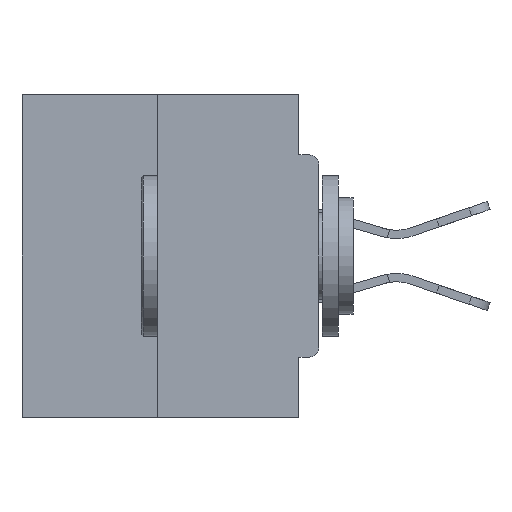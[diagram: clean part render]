
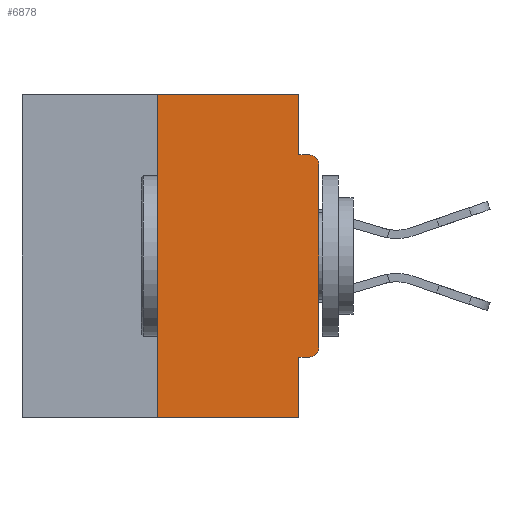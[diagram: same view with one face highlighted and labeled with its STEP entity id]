
A CAD part, left-side view. The second image highlights one B-rep face of the part: STEP entity #6878.
In plain terms, the highlighted planar face has unit normal (-1, 0, 0).
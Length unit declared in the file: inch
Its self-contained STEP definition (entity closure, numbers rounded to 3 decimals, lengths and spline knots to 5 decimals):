
#933 = DIRECTION ( 'NONE',  ( 0., 0., -1. ) ) ;
#1001 = EDGE_CURVE ( 'NONE', #25454, #25395, #29724, .T. ) ;
#1722 = CARTESIAN_POINT ( 'NONE',  ( 0., 0.25, -0.5 ) ) ;
#2146 = ORIENTED_EDGE ( 'NONE', *, *, #30901, .F. ) ;
#3434 = CARTESIAN_POINT ( 'NONE',  ( 0., 0.031, -0.4065 ) ) ;
#4298 = EDGE_LOOP ( 'NONE', ( #2146, #37162, #21792, #23008, #35223, #9632, #7834, #28525, #21918, #13976 ) ) ;
#4309 = DIRECTION ( 'NONE',  ( 0., 0., 1. ) ) ;
#4375 = CARTESIAN_POINT ( 'NONE',  ( 0., 0.25, 0. ) ) ;
#4408 = VERTEX_POINT ( 'NONE', #17975 ) ;
#4445 = EDGE_CURVE ( 'NONE', #8649, #29275, #18057, .T. ) ;
#5433 = LINE ( 'NONE', #18613, #16740 ) ;
#6863 = DIRECTION ( 'NONE',  ( 0., 0., -1. ) ) ;
#6878 = ADVANCED_FACE ( 'NONE', ( #32872 ), #21209, .F. ) ;
#7069 = VECTOR ( 'NONE', #36921, 39.37008 ) ;
#7736 = EDGE_CURVE ( 'NONE', #29275, #28448, #27808, .T. ) ;
#7834 = ORIENTED_EDGE ( 'NONE', *, *, #4445, .T. ) ;
#8486 = LINE ( 'NONE', #9154, #25221 ) ;
#8614 = EDGE_CURVE ( 'NONE', #33012, #25261, #8486, .T. ) ;
#8649 = VERTEX_POINT ( 'NONE', #24083 ) ;
#9154 = CARTESIAN_POINT ( 'NONE',  ( 0., 0., -0.4065 ) ) ;
#9389 = CARTESIAN_POINT ( 'NONE',  ( 0., 0.015, -0.1085 ) ) ;
#9483 = LINE ( 'NONE', #33448, #35346 ) ;
#9632 = ORIENTED_EDGE ( 'NONE', *, *, #24973, .T. ) ;
#10606 = AXIS2_PLACEMENT_3D ( 'NONE', #9389, #29421, #32572 ) ;
#11054 = CARTESIAN_POINT ( 'NONE',  ( 0., 0.25, 0. ) ) ;
#11747 = VECTOR ( 'NONE', #4309, 39.37008 ) ;
#11888 = VECTOR ( 'NONE', #32678, 39.37008 ) ;
#13976 = ORIENTED_EDGE ( 'NONE', *, *, #22977, .F. ) ;
#14160 = CARTESIAN_POINT ( 'NONE',  ( 0., 0.031, -0.5 ) ) ;
#14330 = DIRECTION ( 'NONE',  ( 0., -1., 0. ) ) ;
#15094 = CARTESIAN_POINT ( 'NONE',  ( 0., 0.46, 0. ) ) ;
#15231 = VERTEX_POINT ( 'NONE', #4375 ) ;
#16740 = VECTOR ( 'NONE', #6863, 39.37008 ) ;
#17073 = CARTESIAN_POINT ( 'NONE',  ( 0., 0.015, -0.0935 ) ) ;
#17439 = VECTOR ( 'NONE', #22399, 39.37008 ) ;
#17901 = DIRECTION ( 'NONE',  ( 0., 1., 0. ) ) ;
#17975 = CARTESIAN_POINT ( 'NONE',  ( 0., 0.031, 0. ) ) ;
#18057 = LINE ( 'NONE', #36102, #11747 ) ;
#18613 = CARTESIAN_POINT ( 'NONE',  ( 0., 0.031, 0. ) ) ;
#19743 = VERTEX_POINT ( 'NONE', #37379 ) ;
#21209 = PLANE ( 'NONE',  #28307 ) ;
#21332 = CARTESIAN_POINT ( 'NONE',  ( 0., 0.46, 0. ) ) ;
#21459 = DIRECTION ( 'NONE',  ( 0., 0., -1. ) ) ;
#21792 = ORIENTED_EDGE ( 'NONE', *, *, #1001, .T. ) ;
#21918 = ORIENTED_EDGE ( 'NONE', *, *, #28853, .F. ) ;
#22145 = CARTESIAN_POINT ( 'NONE',  ( 0., 0.46, -0.5 ) ) ;
#22399 = DIRECTION ( 'NONE',  ( 0., -1., 0. ) ) ;
#22406 = VECTOR ( 'NONE', #14330, 39.37008 ) ;
#22455 = CIRCLE ( 'NONE', #28461, 0.015 ) ;
#22977 = EDGE_CURVE ( 'NONE', #4408, #19743, #5433, .T. ) ;
#23008 = ORIENTED_EDGE ( 'NONE', *, *, #23140, .F. ) ;
#23140 = EDGE_CURVE ( 'NONE', #25261, #25395, #9483, .T. ) ;
#24083 = CARTESIAN_POINT ( 'NONE',  ( 0., 0., -0.3915 ) ) ;
#24303 = CARTESIAN_POINT ( 'NONE',  ( 0., 0., -0.1085 ) ) ;
#24688 = DIRECTION ( 'NONE',  ( 0., 0., -1. ) ) ;
#24869 = EDGE_CURVE ( 'NONE', #25454, #15231, #31101, .T. ) ;
#24973 = EDGE_CURVE ( 'NONE', #33012, #8649, #22455, .T. ) ;
#25221 = VECTOR ( 'NONE', #17901, 39.37008 ) ;
#25261 = VERTEX_POINT ( 'NONE', #3434 ) ;
#25395 = VERTEX_POINT ( 'NONE', #14160 ) ;
#25454 = VERTEX_POINT ( 'NONE', #1722 ) ;
#27808 = CIRCLE ( 'NONE', #10606, 0.015 ) ;
#28307 = AXIS2_PLACEMENT_3D ( 'NONE', #21332, #32734, #21459 ) ;
#28448 = VERTEX_POINT ( 'NONE', #17073 ) ;
#28461 = AXIS2_PLACEMENT_3D ( 'NONE', #29678, #35494, #933 ) ;
#28525 = ORIENTED_EDGE ( 'NONE', *, *, #7736, .T. ) ;
#28656 = LINE ( 'NONE', #15094, #11888 ) ;
#28853 = EDGE_CURVE ( 'NONE', #19743, #28448, #37403, .T. ) ;
#29275 = VERTEX_POINT ( 'NONE', #24303 ) ;
#29421 = DIRECTION ( 'NONE',  ( -1., 0., 0. ) ) ;
#29678 = CARTESIAN_POINT ( 'NONE',  ( 0., 0.015, -0.3915 ) ) ;
#29724 = LINE ( 'NONE', #22145, #17439 ) ;
#30901 = EDGE_CURVE ( 'NONE', #15231, #4408, #28656, .T. ) ;
#31101 = LINE ( 'NONE', #11054, #7069 ) ;
#32572 = DIRECTION ( 'NONE',  ( 0., 0., -1. ) ) ;
#32678 = DIRECTION ( 'NONE',  ( 0., -1., 0. ) ) ;
#32734 = DIRECTION ( 'NONE',  ( 1., 0., 0. ) ) ;
#32872 = FACE_OUTER_BOUND ( 'NONE', #4298, .T. ) ;
#33012 = VERTEX_POINT ( 'NONE', #34735 ) ;
#33448 = CARTESIAN_POINT ( 'NONE',  ( 0., 0.031, -0.5 ) ) ;
#34238 = CARTESIAN_POINT ( 'NONE',  ( 0., 0., -0.0935 ) ) ;
#34735 = CARTESIAN_POINT ( 'NONE',  ( 0., 0.015, -0.4065 ) ) ;
#35223 = ORIENTED_EDGE ( 'NONE', *, *, #8614, .F. ) ;
#35346 = VECTOR ( 'NONE', #24688, 39.37008 ) ;
#35494 = DIRECTION ( 'NONE',  ( -1., 0., 0. ) ) ;
#36102 = CARTESIAN_POINT ( 'NONE',  ( 0., 0., 0. ) ) ;
#36921 = DIRECTION ( 'NONE',  ( 0., 0., 1. ) ) ;
#37162 = ORIENTED_EDGE ( 'NONE', *, *, #24869, .F. ) ;
#37379 = CARTESIAN_POINT ( 'NONE',  ( 0., 0.031, -0.0935 ) ) ;
#37403 = LINE ( 'NONE', #34238, #22406 ) ;
